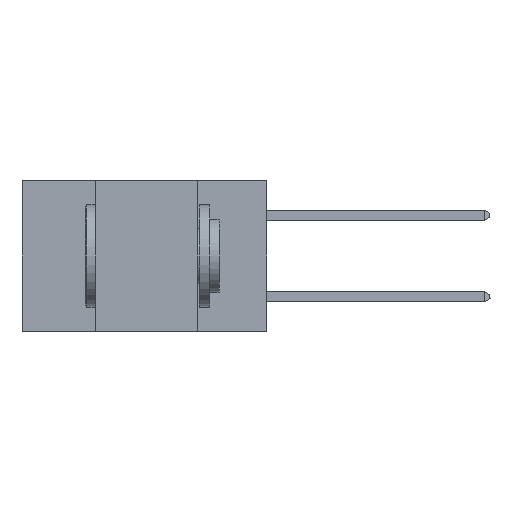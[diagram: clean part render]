
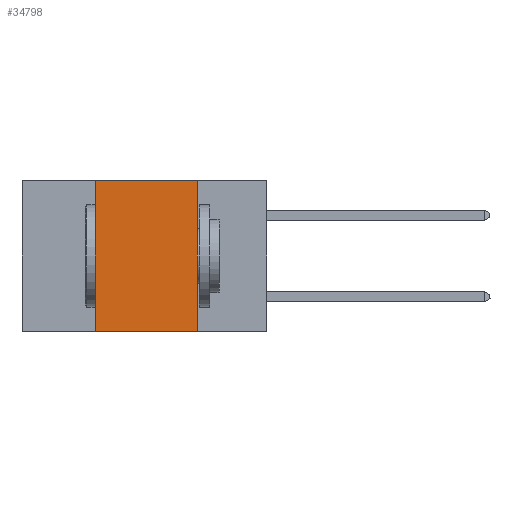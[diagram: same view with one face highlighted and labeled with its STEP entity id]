
A CAD part, left-side view. The second image highlights one B-rep face of the part: STEP entity #34798.
In plain terms, the highlighted planar face has unit normal (-1, 0, 0).
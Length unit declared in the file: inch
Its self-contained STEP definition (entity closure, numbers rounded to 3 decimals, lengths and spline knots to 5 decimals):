
#360 = CARTESIAN_POINT ( 'NONE',  ( 0., 0.6, 0. ) ) ;
#539 = VECTOR ( 'NONE', #31700, 39.37008 ) ;
#599 = LINE ( 'NONE', #11748, #36834 ) ;
#3530 = PLANE ( 'NONE',  #24590 ) ;
#4078 = VECTOR ( 'NONE', #14815, 39.37008 ) ;
#4979 = LINE ( 'NONE', #360, #4078 ) ;
#7239 = EDGE_CURVE ( 'NONE', #24509, #22426, #599, .T. ) ;
#8408 = CARTESIAN_POINT ( 'NONE',  ( 0., 0.17, -0.37 ) ) ;
#8842 = CARTESIAN_POINT ( 'NONE',  ( 0., 0.42, 0. ) ) ;
#11549 = EDGE_CURVE ( 'NONE', #28630, #22426, #35201, .T. ) ;
#11748 = CARTESIAN_POINT ( 'NONE',  ( 0., 0.6, -0.37 ) ) ;
#11772 = CARTESIAN_POINT ( 'NONE',  ( 0., 0.42, -0.37 ) ) ;
#12364 = ORIENTED_EDGE ( 'NONE', *, *, #26313, .F. ) ;
#14161 = EDGE_CURVE ( 'NONE', #24509, #26871, #15852, .T. ) ;
#14265 = CARTESIAN_POINT ( 'NONE',  ( 0., 0.42, 0. ) ) ;
#14705 = CARTESIAN_POINT ( 'NONE',  ( 0., 0.17, 0. ) ) ;
#14815 = DIRECTION ( 'NONE',  ( 0., -1., 0. ) ) ;
#15045 = CARTESIAN_POINT ( 'NONE',  ( 0., 0.6, 0. ) ) ;
#15178 = DIRECTION ( 'NONE',  ( 1., 0., 0. ) ) ;
#15852 = LINE ( 'NONE', #8842, #539 ) ;
#18162 = ORIENTED_EDGE ( 'NONE', *, *, #11549, .F. ) ;
#19984 = ORIENTED_EDGE ( 'NONE', *, *, #14161, .F. ) ;
#20498 = DIRECTION ( 'NONE',  ( 0., 0., -1. ) ) ;
#22426 = VERTEX_POINT ( 'NONE', #8408 ) ;
#24509 = VERTEX_POINT ( 'NONE', #11772 ) ;
#24590 = AXIS2_PLACEMENT_3D ( 'NONE', #15045, #15178, #35106 ) ;
#26313 = EDGE_CURVE ( 'NONE', #26871, #28630, #4979, .T. ) ;
#26871 = VERTEX_POINT ( 'NONE', #14265 ) ;
#27702 = VECTOR ( 'NONE', #20498, 39.37008 ) ;
#28630 = VERTEX_POINT ( 'NONE', #34289 ) ;
#28919 = DIRECTION ( 'NONE',  ( 0., -1., 0. ) ) ;
#30527 = FACE_OUTER_BOUND ( 'NONE', #35492, .T. ) ;
#31700 = DIRECTION ( 'NONE',  ( 0., 0., 1. ) ) ;
#34289 = CARTESIAN_POINT ( 'NONE',  ( 0., 0.17, 0. ) ) ;
#34798 = ADVANCED_FACE ( 'NONE', ( #30527 ), #3530, .F. ) ;
#35106 = DIRECTION ( 'NONE',  ( 0., 0., -1. ) ) ;
#35201 = LINE ( 'NONE', #14705, #27702 ) ;
#35492 = EDGE_LOOP ( 'NONE', ( #18162, #12364, #19984, #35977 ) ) ;
#35977 = ORIENTED_EDGE ( 'NONE', *, *, #7239, .T. ) ;
#36834 = VECTOR ( 'NONE', #28919, 39.37008 ) ;
